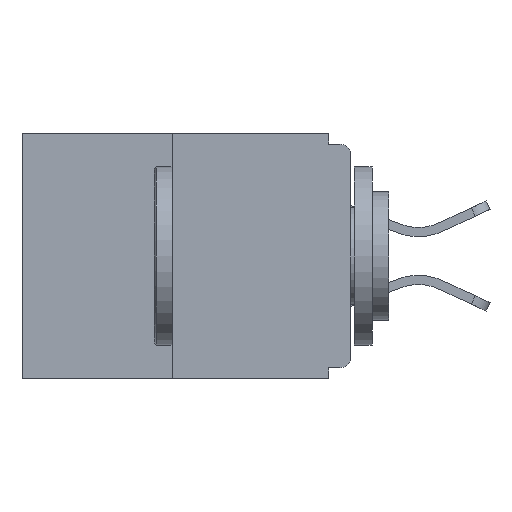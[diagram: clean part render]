
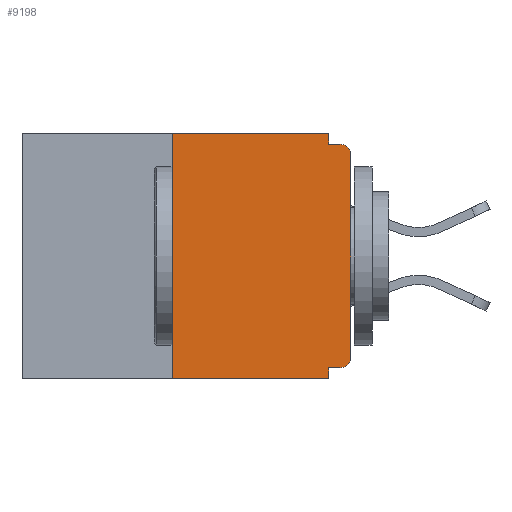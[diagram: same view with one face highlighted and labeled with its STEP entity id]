
A CAD part, left-side view. The second image highlights one B-rep face of the part: STEP entity #9198.
In plain terms, the highlighted planar face has unit normal (-1, 0, 0).
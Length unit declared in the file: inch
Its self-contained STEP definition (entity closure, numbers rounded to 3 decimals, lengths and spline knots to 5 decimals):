
#320 = CARTESIAN_POINT ( 'NONE',  ( 0., 0.015, -0.03 ) ) ;
#346 = LINE ( 'NONE', #19606, #15899 ) ;
#499 = LINE ( 'NONE', #20224, #18829 ) ;
#640 = AXIS2_PLACEMENT_3D ( 'NONE', #11540, #1904, #13179 ) ;
#657 = CARTESIAN_POINT ( 'NONE',  ( 0., 0.031, 0. ) ) ;
#1110 = VECTOR ( 'NONE', #12248, 39.37008 ) ;
#1437 = CARTESIAN_POINT ( 'NONE',  ( 0., 0.031, -0.328 ) ) ;
#1589 = EDGE_CURVE ( 'NONE', #12226, #19161, #10240, .T. ) ;
#1896 = LINE ( 'NONE', #6545, #14229 ) ;
#1904 = DIRECTION ( 'NONE',  ( 1., 0., 0. ) ) ;
#2051 = AXIS2_PLACEMENT_3D ( 'NONE', #6458, #3420, #11511 ) ;
#2066 = DIRECTION ( 'NONE',  ( -1., 0., 0. ) ) ;
#3085 = VERTEX_POINT ( 'NONE', #11739 ) ;
#3116 = VERTEX_POINT ( 'NONE', #19472 ) ;
#3420 = DIRECTION ( 'NONE',  ( -1., 0., 0. ) ) ;
#3531 = VERTEX_POINT ( 'NONE', #5990 ) ;
#4026 = EDGE_CURVE ( 'NONE', #11847, #16629, #20772, .T. ) ;
#4074 = VECTOR ( 'NONE', #16513, 39.37008 ) ;
#4126 = DIRECTION ( 'NONE',  ( 0., 1., 0. ) ) ;
#4504 = EDGE_CURVE ( 'NONE', #12226, #11847, #12729, .T. ) ;
#4929 = DIRECTION ( 'NONE',  ( 0., 0., 1. ) ) ;
#4993 = VERTEX_POINT ( 'NONE', #5618 ) ;
#5213 = ORIENTED_EDGE ( 'NONE', *, *, #18184, .T. ) ;
#5272 = CIRCLE ( 'NONE', #7432, 0.015 ) ;
#5410 = LINE ( 'NONE', #12454, #1110 ) ;
#5604 = EDGE_CURVE ( 'NONE', #3531, #3116, #1896, .T. ) ;
#5618 = CARTESIAN_POINT ( 'NONE',  ( 0., 0.25, -0.343 ) ) ;
#5990 = CARTESIAN_POINT ( 'NONE',  ( 0., 0.031, -0.015 ) ) ;
#6458 = CARTESIAN_POINT ( 'NONE',  ( 0., 0.015, -0.313 ) ) ;
#6545 = CARTESIAN_POINT ( 'NONE',  ( 0., 0., -0.015 ) ) ;
#7253 = CARTESIAN_POINT ( 'NONE',  ( 0., 0., -0.313 ) ) ;
#7394 = CARTESIAN_POINT ( 'NONE',  ( 0., 0.46, -0.343 ) ) ;
#7432 = AXIS2_PLACEMENT_3D ( 'NONE', #320, #2066, #11638 ) ;
#7485 = VECTOR ( 'NONE', #4126, 39.37008 ) ;
#7546 = ORIENTED_EDGE ( 'NONE', *, *, #8585, .F. ) ;
#8520 = ORIENTED_EDGE ( 'NONE', *, *, #14841, .F. ) ;
#8585 = EDGE_CURVE ( 'NONE', #19161, #15560, #499, .T. ) ;
#8989 = EDGE_LOOP ( 'NONE', ( #13686, #20182, #5213, #7546, #11292, #17769, #16262, #14264, #13099, #8520 ) ) ;
#9198 = ADVANCED_FACE ( 'NONE', ( #15792 ), #19552, .F. ) ;
#10240 = LINE ( 'NONE', #20195, #7485 ) ;
#11283 = EDGE_CURVE ( 'NONE', #16629, #3116, #5272, .T. ) ;
#11292 = ORIENTED_EDGE ( 'NONE', *, *, #1589, .F. ) ;
#11511 = DIRECTION ( 'NONE',  ( 0., 0., -1. ) ) ;
#11540 = CARTESIAN_POINT ( 'NONE',  ( 0., 0.46, 0. ) ) ;
#11638 = DIRECTION ( 'NONE',  ( 0., 0., -1. ) ) ;
#11739 = CARTESIAN_POINT ( 'NONE',  ( 0., 0.25, 0. ) ) ;
#11847 = VERTEX_POINT ( 'NONE', #7253 ) ;
#12226 = VERTEX_POINT ( 'NONE', #16693 ) ;
#12248 = DIRECTION ( 'NONE',  ( 0., -1., 0. ) ) ;
#12454 = CARTESIAN_POINT ( 'NONE',  ( 0., 0.46, 0. ) ) ;
#12729 = CIRCLE ( 'NONE', #2051, 0.015 ) ;
#13099 = ORIENTED_EDGE ( 'NONE', *, *, #5604, .F. ) ;
#13179 = DIRECTION ( 'NONE',  ( 0., 0., -1. ) ) ;
#13289 = DIRECTION ( 'NONE',  ( 0., 0., -1. ) ) ;
#13504 = CARTESIAN_POINT ( 'NONE',  ( 0., 0.25, 0. ) ) ;
#13587 = VECTOR ( 'NONE', #19179, 39.37008 ) ;
#13686 = ORIENTED_EDGE ( 'NONE', *, *, #13699, .F. ) ;
#13699 = EDGE_CURVE ( 'NONE', #3085, #13998, #5410, .T. ) ;
#13998 = VERTEX_POINT ( 'NONE', #657 ) ;
#14229 = VECTOR ( 'NONE', #19265, 39.37008 ) ;
#14264 = ORIENTED_EDGE ( 'NONE', *, *, #11283, .T. ) ;
#14403 = LINE ( 'NONE', #13504, #4074 ) ;
#14841 = EDGE_CURVE ( 'NONE', #13998, #3531, #346, .T. ) ;
#15560 = VERTEX_POINT ( 'NONE', #16288 ) ;
#15792 = FACE_OUTER_BOUND ( 'NONE', #8989, .T. ) ;
#15899 = VECTOR ( 'NONE', #13289, 39.37008 ) ;
#16262 = ORIENTED_EDGE ( 'NONE', *, *, #4026, .T. ) ;
#16288 = CARTESIAN_POINT ( 'NONE',  ( 0., 0.031, -0.343 ) ) ;
#16513 = DIRECTION ( 'NONE',  ( 0., 0., 1. ) ) ;
#16520 = VECTOR ( 'NONE', #4929, 39.37008 ) ;
#16629 = VERTEX_POINT ( 'NONE', #20271 ) ;
#16693 = CARTESIAN_POINT ( 'NONE',  ( 0., 0.015, -0.328 ) ) ;
#16869 = DIRECTION ( 'NONE',  ( 0., 0., -1. ) ) ;
#17769 = ORIENTED_EDGE ( 'NONE', *, *, #4504, .T. ) ;
#18184 = EDGE_CURVE ( 'NONE', #4993, #15560, #18365, .T. ) ;
#18365 = LINE ( 'NONE', #7394, #13587 ) ;
#18829 = VECTOR ( 'NONE', #16869, 39.37008 ) ;
#19161 = VERTEX_POINT ( 'NONE', #1437 ) ;
#19179 = DIRECTION ( 'NONE',  ( 0., -1., 0. ) ) ;
#19265 = DIRECTION ( 'NONE',  ( 0., -1., 0. ) ) ;
#19472 = CARTESIAN_POINT ( 'NONE',  ( 0., 0.015, -0.015 ) ) ;
#19552 = PLANE ( 'NONE',  #640 ) ;
#19606 = CARTESIAN_POINT ( 'NONE',  ( 0., 0.031, 0. ) ) ;
#19958 = EDGE_CURVE ( 'NONE', #4993, #3085, #14403, .T. ) ;
#20182 = ORIENTED_EDGE ( 'NONE', *, *, #19958, .F. ) ;
#20195 = CARTESIAN_POINT ( 'NONE',  ( 0., 0., -0.328 ) ) ;
#20224 = CARTESIAN_POINT ( 'NONE',  ( 0., 0.031, -0.343 ) ) ;
#20271 = CARTESIAN_POINT ( 'NONE',  ( 0., 0., -0.03 ) ) ;
#20374 = CARTESIAN_POINT ( 'NONE',  ( 0., 0., 0. ) ) ;
#20772 = LINE ( 'NONE', #20374, #16520 ) ;
